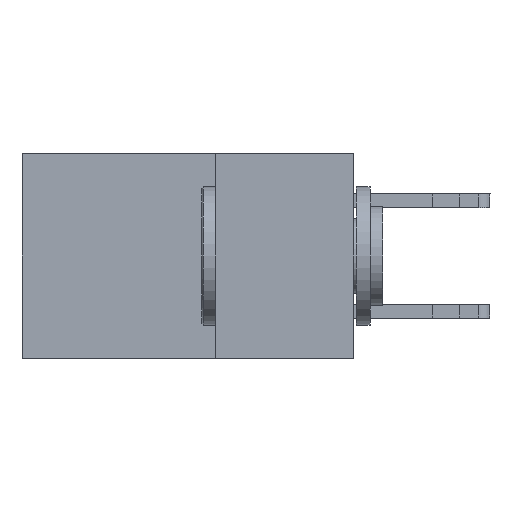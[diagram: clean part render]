
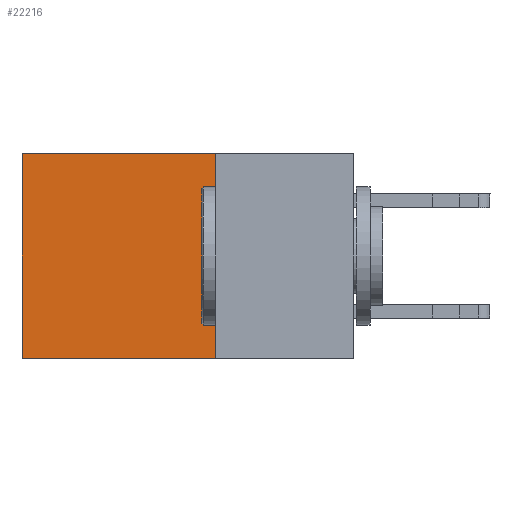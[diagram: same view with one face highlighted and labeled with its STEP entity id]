
A CAD part, left-side view. The second image highlights one B-rep face of the part: STEP entity #22216.
In plain terms, the highlighted planar face has unit normal (-1, 0, 0).
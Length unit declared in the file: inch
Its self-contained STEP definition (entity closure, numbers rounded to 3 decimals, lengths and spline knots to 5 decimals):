
#269 = VERTEX_POINT ( 'NONE', #13668 ) ;
#1299 = DIRECTION ( 'NONE',  ( 0., 1., 0. ) ) ;
#1615 = EDGE_LOOP ( 'NONE', ( #9651, #14627, #5669, #35251 ) ) ;
#1723 = VECTOR ( 'NONE', #26820, 39.37008 ) ;
#3389 = PLANE ( 'NONE',  #26415 ) ;
#3588 = CARTESIAN_POINT ( 'NONE',  ( 0.2875, 0.25, 0. ) ) ;
#4056 = CARTESIAN_POINT ( 'NONE',  ( 0.2875, 0.25, -0.37 ) ) ;
#4705 = VECTOR ( 'NONE', #28988, 39.37008 ) ;
#5099 = CARTESIAN_POINT ( 'NONE',  ( 0.2875, 0.6, -0.37 ) ) ;
#5669 = ORIENTED_EDGE ( 'NONE', *, *, #16526, .F. ) ;
#6994 = EDGE_CURVE ( 'NONE', #34372, #269, #24918, .T. ) ;
#7422 = VECTOR ( 'NONE', #16784, 39.37008 ) ;
#8933 = CARTESIAN_POINT ( 'NONE',  ( 0.2875, 0.25, 0. ) ) ;
#9651 = ORIENTED_EDGE ( 'NONE', *, *, #15731, .T. ) ;
#12383 = LINE ( 'NONE', #30892, #7422 ) ;
#13668 = CARTESIAN_POINT ( 'NONE',  ( 0.2875, 0.6, 0. ) ) ;
#14627 = ORIENTED_EDGE ( 'NONE', *, *, #23667, .F. ) ;
#14673 = CARTESIAN_POINT ( 'NONE',  ( 0.2875, 0.25, 0. ) ) ;
#15731 = EDGE_CURVE ( 'NONE', #269, #26073, #12383, .T. ) ;
#16526 = EDGE_CURVE ( 'NONE', #34372, #24229, #19936, .T. ) ;
#16784 = DIRECTION ( 'NONE',  ( 0., 0., -1. ) ) ;
#19936 = LINE ( 'NONE', #29220, #4705 ) ;
#21207 = DIRECTION ( 'NONE',  ( 0., 0., -1. ) ) ;
#22216 = ADVANCED_FACE ( 'NONE', ( #22390 ), #3389, .F. ) ;
#22390 = FACE_OUTER_BOUND ( 'NONE', #1615, .T. ) ;
#23315 = DIRECTION ( 'NONE',  ( 1., 0., 0. ) ) ;
#23667 = EDGE_CURVE ( 'NONE', #24229, #26073, #31172, .T. ) ;
#24229 = VERTEX_POINT ( 'NONE', #34485 ) ;
#24918 = LINE ( 'NONE', #3588, #32426 ) ;
#26073 = VERTEX_POINT ( 'NONE', #5099 ) ;
#26415 = AXIS2_PLACEMENT_3D ( 'NONE', #14673, #23315, #21207 ) ;
#26820 = DIRECTION ( 'NONE',  ( 0., 1., 0. ) ) ;
#28988 = DIRECTION ( 'NONE',  ( 0., 0., -1. ) ) ;
#29220 = CARTESIAN_POINT ( 'NONE',  ( 0.2875, 0.25, 0. ) ) ;
#30892 = CARTESIAN_POINT ( 'NONE',  ( 0.2875, 0.6, 0. ) ) ;
#31172 = LINE ( 'NONE', #4056, #1723 ) ;
#32426 = VECTOR ( 'NONE', #1299, 39.37008 ) ;
#34372 = VERTEX_POINT ( 'NONE', #8933 ) ;
#34485 = CARTESIAN_POINT ( 'NONE',  ( 0.2875, 0.25, -0.37 ) ) ;
#35251 = ORIENTED_EDGE ( 'NONE', *, *, #6994, .T. ) ;
